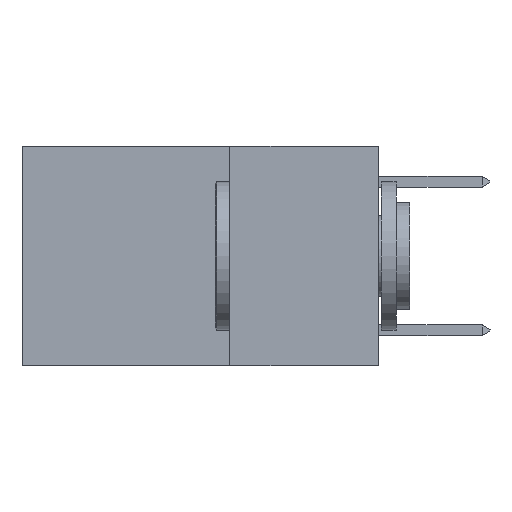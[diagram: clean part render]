
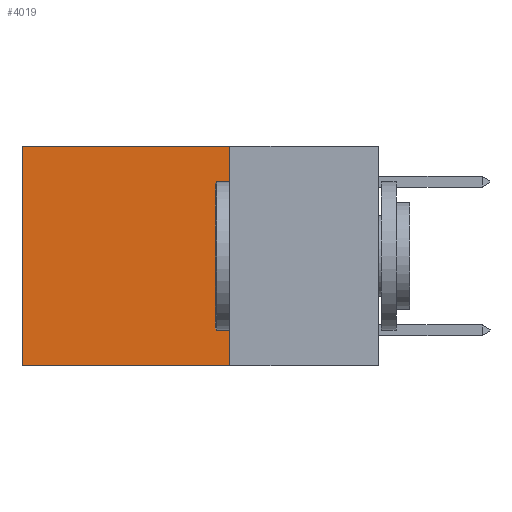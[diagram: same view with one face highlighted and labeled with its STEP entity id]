
A CAD part, left-side view. The second image highlights one B-rep face of the part: STEP entity #4019.
In plain terms, the highlighted planar face has unit normal (-1, 0, 0).
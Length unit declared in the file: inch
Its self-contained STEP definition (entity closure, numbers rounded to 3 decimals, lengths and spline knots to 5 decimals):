
#205 = ORIENTED_EDGE ( 'NONE', *, *, #4023, .T. ) ;
#518 = CARTESIAN_POINT ( 'NONE',  ( 0.2625, 0.6, -0.37 ) ) ;
#1651 = DIRECTION ( 'NONE',  ( 0., 1., 0. ) ) ;
#1682 = CARTESIAN_POINT ( 'NONE',  ( 0.2625, 0.25, -0.37 ) ) ;
#1784 = ORIENTED_EDGE ( 'NONE', *, *, #2008, .F. ) ;
#2008 = EDGE_CURVE ( 'NONE', #2993, #10213, #10434, .T. ) ;
#2179 = EDGE_CURVE ( 'NONE', #8952, #2993, #7247, .T. ) ;
#2437 = CARTESIAN_POINT ( 'NONE',  ( 0.2625, 0.25, 0. ) ) ;
#2597 = EDGE_LOOP ( 'NONE', ( #9227, #1784, #9835, #205 ) ) ;
#2599 = DIRECTION ( 'NONE',  ( 0., 1., 0. ) ) ;
#2712 = VERTEX_POINT ( 'NONE', #6461 ) ;
#2898 = AXIS2_PLACEMENT_3D ( 'NONE', #4311, #8378, #5986 ) ;
#2986 = CARTESIAN_POINT ( 'NONE',  ( 0.2625, 0.25, -0.37 ) ) ;
#2993 = VERTEX_POINT ( 'NONE', #2986 ) ;
#4019 = ADVANCED_FACE ( 'NONE', ( #8512 ), #5162, .F. ) ;
#4023 = EDGE_CURVE ( 'NONE', #8952, #2712, #6099, .T. ) ;
#4143 = VECTOR ( 'NONE', #2599, 39.37008 ) ;
#4194 = VECTOR ( 'NONE', #1651, 39.37008 ) ;
#4311 = CARTESIAN_POINT ( 'NONE',  ( 0.2625, 0.25, 0. ) ) ;
#5123 = VECTOR ( 'NONE', #9602, 39.37008 ) ;
#5162 = PLANE ( 'NONE',  #2898 ) ;
#5986 = DIRECTION ( 'NONE',  ( 0., 0., -1. ) ) ;
#6099 = LINE ( 'NONE', #7581, #4143 ) ;
#6461 = CARTESIAN_POINT ( 'NONE',  ( 0.2625, 0.6, 0. ) ) ;
#7247 = LINE ( 'NONE', #2437, #5123 ) ;
#7255 = CARTESIAN_POINT ( 'NONE',  ( 0.2625, 0.6, 0. ) ) ;
#7581 = CARTESIAN_POINT ( 'NONE',  ( 0.2625, 0.25, 0. ) ) ;
#8065 = LINE ( 'NONE', #7255, #9991 ) ;
#8085 = DIRECTION ( 'NONE',  ( 0., 0., -1. ) ) ;
#8378 = DIRECTION ( 'NONE',  ( 1., 0., 0. ) ) ;
#8512 = FACE_OUTER_BOUND ( 'NONE', #2597, .T. ) ;
#8906 = EDGE_CURVE ( 'NONE', #2712, #10213, #8065, .T. ) ;
#8952 = VERTEX_POINT ( 'NONE', #8967 ) ;
#8967 = CARTESIAN_POINT ( 'NONE',  ( 0.2625, 0.25, 0. ) ) ;
#9227 = ORIENTED_EDGE ( 'NONE', *, *, #8906, .T. ) ;
#9602 = DIRECTION ( 'NONE',  ( 0., 0., -1. ) ) ;
#9835 = ORIENTED_EDGE ( 'NONE', *, *, #2179, .F. ) ;
#9991 = VECTOR ( 'NONE', #8085, 39.37008 ) ;
#10213 = VERTEX_POINT ( 'NONE', #518 ) ;
#10434 = LINE ( 'NONE', #1682, #4194 ) ;
